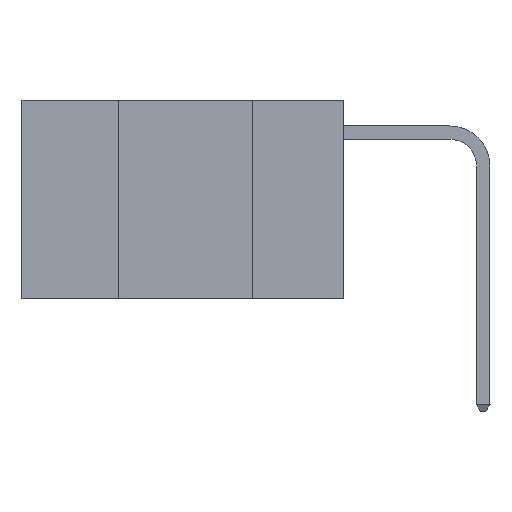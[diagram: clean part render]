
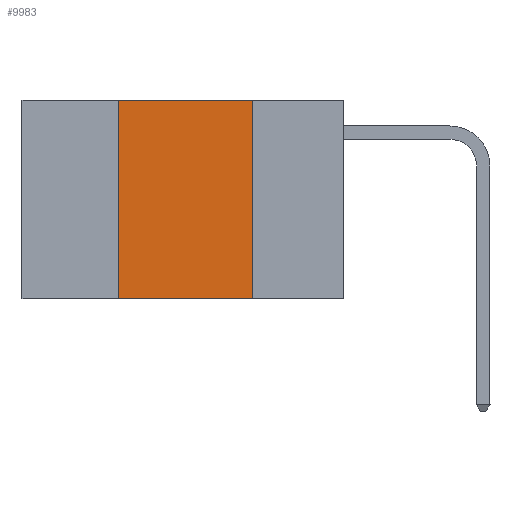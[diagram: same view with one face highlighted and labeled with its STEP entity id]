
A CAD part, left-side view. The second image highlights one B-rep face of the part: STEP entity #9983.
In plain terms, the highlighted planar face has unit normal (-1, 0, 0).
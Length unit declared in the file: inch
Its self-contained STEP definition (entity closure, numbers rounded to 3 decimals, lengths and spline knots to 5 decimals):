
#1023 = CARTESIAN_POINT ( 'NONE',  ( 0., 0.42, 0. ) ) ;
#1083 = DIRECTION ( 'NONE',  ( 0., -1., 0. ) ) ;
#2143 = CARTESIAN_POINT ( 'NONE',  ( 0., 0.6, -0.37 ) ) ;
#2666 = CARTESIAN_POINT ( 'NONE',  ( 0., 0.42, -0.37 ) ) ;
#3356 = LINE ( 'NONE', #2143, #16377 ) ;
#4060 = PLANE ( 'NONE',  #11572 ) ;
#4196 = ORIENTED_EDGE ( 'NONE', *, *, #6299, .F. ) ;
#4398 = ORIENTED_EDGE ( 'NONE', *, *, #16406, .F. ) ;
#4418 = ORIENTED_EDGE ( 'NONE', *, *, #15596, .F. ) ;
#4636 = ORIENTED_EDGE ( 'NONE', *, *, #13213, .T. ) ;
#4848 = DIRECTION ( 'NONE',  ( 0., 0., 1. ) ) ;
#6153 = VERTEX_POINT ( 'NONE', #1023 ) ;
#6299 = EDGE_CURVE ( 'NONE', #7414, #15642, #14906, .T. ) ;
#6566 = LINE ( 'NONE', #12390, #16099 ) ;
#6646 = CARTESIAN_POINT ( 'NONE',  ( 0., 0.17, 0. ) ) ;
#7414 = VERTEX_POINT ( 'NONE', #7560 ) ;
#7560 = CARTESIAN_POINT ( 'NONE',  ( 0., 0.17, 0. ) ) ;
#8720 = CARTESIAN_POINT ( 'NONE',  ( 0., 0.17, -0.37 ) ) ;
#9167 = DIRECTION ( 'NONE',  ( 1., 0., 0. ) ) ;
#9453 = VERTEX_POINT ( 'NONE', #2666 ) ;
#9856 = VECTOR ( 'NONE', #1083, 39.37008 ) ;
#9983 = ADVANCED_FACE ( 'NONE', ( #16152 ), #4060, .F. ) ;
#11037 = DIRECTION ( 'NONE',  ( 0., 0., -1. ) ) ;
#11572 = AXIS2_PLACEMENT_3D ( 'NONE', #14130, #9167, #11037 ) ;
#11620 = VECTOR ( 'NONE', #15364, 39.37008 ) ;
#12390 = CARTESIAN_POINT ( 'NONE',  ( 0., 0.42, 0. ) ) ;
#13187 = LINE ( 'NONE', #15027, #9856 ) ;
#13213 = EDGE_CURVE ( 'NONE', #9453, #15642, #3356, .T. ) ;
#13586 = DIRECTION ( 'NONE',  ( 0., -1., 0. ) ) ;
#14130 = CARTESIAN_POINT ( 'NONE',  ( 0., 0.6, 0. ) ) ;
#14856 = EDGE_LOOP ( 'NONE', ( #4196, #4398, #4418, #4636 ) ) ;
#14906 = LINE ( 'NONE', #6646, #11620 ) ;
#15027 = CARTESIAN_POINT ( 'NONE',  ( 0., 0.6, 0. ) ) ;
#15364 = DIRECTION ( 'NONE',  ( 0., 0., -1. ) ) ;
#15596 = EDGE_CURVE ( 'NONE', #9453, #6153, #6566, .T. ) ;
#15642 = VERTEX_POINT ( 'NONE', #8720 ) ;
#16099 = VECTOR ( 'NONE', #4848, 39.37008 ) ;
#16152 = FACE_OUTER_BOUND ( 'NONE', #14856, .T. ) ;
#16377 = VECTOR ( 'NONE', #13586, 39.37008 ) ;
#16406 = EDGE_CURVE ( 'NONE', #6153, #7414, #13187, .T. ) ;
